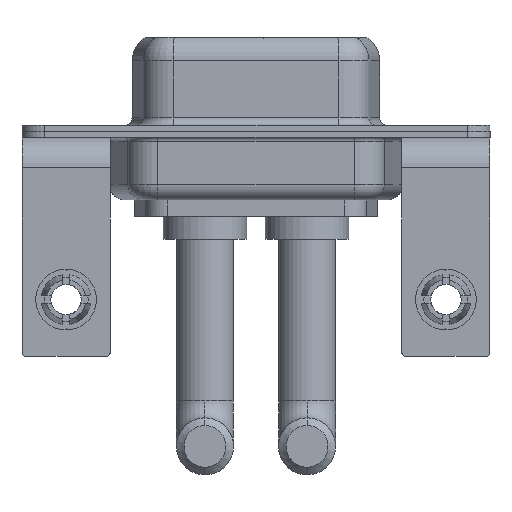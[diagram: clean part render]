
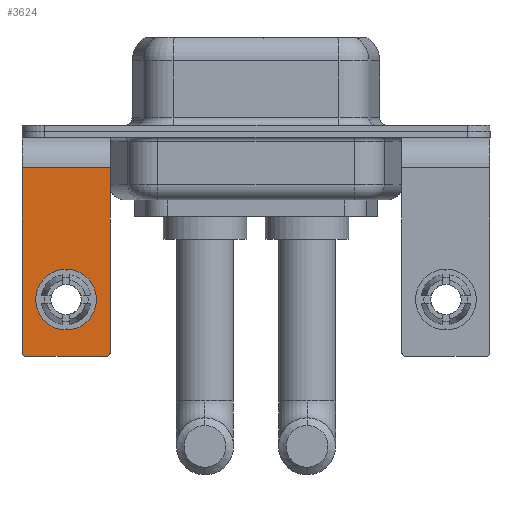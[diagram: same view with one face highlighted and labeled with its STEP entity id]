
A CAD part, front view. The second image highlights one B-rep face of the part: STEP entity #3624.
In plain terms, the highlighted planar face has unit normal (0, -1, 0).
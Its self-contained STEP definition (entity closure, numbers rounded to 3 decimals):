
#23 = DIRECTION ( 'NONE',  ( 0., 0., 1. ) ) ;
#254 = ORIENTED_EDGE ( 'NONE', *, *, #11016, .T. ) ;
#834 = CARTESIAN_POINT ( 'NONE',  ( 2.9, -6.25, -2.4 ) ) ;
#1071 = DIRECTION ( 'NONE',  ( 0., 1., 0. ) ) ;
#1249 = CARTESIAN_POINT ( 'NONE',  ( 2.65, -6.25, -14.8 ) ) ;
#1402 = CARTESIAN_POINT ( 'NONE',  ( -2.9, -6.25, -14.55 ) ) ;
#1406 = EDGE_CURVE ( 'NONE', #9233, #6474, #4739, .T. ) ;
#2445 = ORIENTED_EDGE ( 'NONE', *, *, #6453, .T. ) ;
#2625 = DIRECTION ( 'NONE',  ( 0., -1., 0. ) ) ;
#2929 = CARTESIAN_POINT ( 'NONE',  ( 0., -6.25, -11.07 ) ) ;
#3060 = CARTESIAN_POINT ( 'NONE',  ( 2.9, -6.25, -14.55 ) ) ;
#3472 = ORIENTED_EDGE ( 'NONE', *, *, #8617, .T. ) ;
#3624 = ADVANCED_FACE ( 'NONE', ( #4878, #4643 ), #10825, .F. ) ;
#3916 = DIRECTION ( 'NONE',  ( 0., 1., 0. ) ) ;
#4448 = ORIENTED_EDGE ( 'NONE', *, *, #8715, .T. ) ;
#4521 = VERTEX_POINT ( 'NONE', #1402 ) ;
#4624 = EDGE_CURVE ( 'NONE', #6474, #9233, #7507, .T. ) ;
#4631 = CARTESIAN_POINT ( 'NONE',  ( 2.65, -6.25, -14.55 ) ) ;
#4643 = FACE_OUTER_BOUND ( 'NONE', #7468, .T. ) ;
#4739 = CIRCLE ( 'NONE', #14375, 2. ) ;
#4878 = FACE_BOUND ( 'NONE', #11897, .T. ) ;
#5662 = EDGE_CURVE ( 'NONE', #8594, #13897, #6390, .T. ) ;
#6112 = AXIS2_PLACEMENT_3D ( 'NONE', #14547, #2625, #23 ) ;
#6349 = VERTEX_POINT ( 'NONE', #1249 ) ;
#6390 = LINE ( 'NONE', #8855, #10854 ) ;
#6453 = EDGE_CURVE ( 'NONE', #6846, #4521, #7923, .T. ) ;
#6474 = VERTEX_POINT ( 'NONE', #8875 ) ;
#6846 = VERTEX_POINT ( 'NONE', #13601 ) ;
#7468 = EDGE_LOOP ( 'NONE', ( #2445, #4448, #9600, #3472, #8025, #254 ) ) ;
#7507 = CIRCLE ( 'NONE', #9537, 2. ) ;
#7571 = DIRECTION ( 'NONE',  ( 0., 1., 0. ) ) ;
#7827 = CARTESIAN_POINT ( 'NONE',  ( 0., -6.25, -11.07 ) ) ;
#7923 = LINE ( 'NONE', #10120, #14914 ) ;
#8025 = ORIENTED_EDGE ( 'NONE', *, *, #5662, .F. ) ;
#8559 = VERTEX_POINT ( 'NONE', #10661 ) ;
#8594 = VERTEX_POINT ( 'NONE', #834 ) ;
#8617 = EDGE_CURVE ( 'NONE', #6349, #13897, #9399, .T. ) ;
#8656 = CIRCLE ( 'NONE', #6112, 0.25 ) ;
#8715 = EDGE_CURVE ( 'NONE', #4521, #8559, #8656, .T. ) ;
#8855 = CARTESIAN_POINT ( 'NONE',  ( 2.9, -6.25, -2.4 ) ) ;
#8875 = CARTESIAN_POINT ( 'NONE',  ( 0., -6.25, -13.07 ) ) ;
#8977 = EDGE_CURVE ( 'NONE', #6349, #8559, #12467, .T. ) ;
#9154 = CARTESIAN_POINT ( 'NONE',  ( 2.9, -6.25, -14.8 ) ) ;
#9233 = VERTEX_POINT ( 'NONE', #12062 ) ;
#9399 = CIRCLE ( 'NONE', #11400, 0.25 ) ;
#9537 = AXIS2_PLACEMENT_3D ( 'NONE', #2929, #7571, #11349 ) ;
#9569 = CARTESIAN_POINT ( 'NONE',  ( 2.9, -6.25, -2.4 ) ) ;
#9600 = ORIENTED_EDGE ( 'NONE', *, *, #8977, .F. ) ;
#10110 = DIRECTION ( 'NONE',  ( 0., 0., 1. ) ) ;
#10120 = CARTESIAN_POINT ( 'NONE',  ( -2.9, -6.25, -2.4 ) ) ;
#10504 = DIRECTION ( 'NONE',  ( 0., 0., 1. ) ) ;
#10562 = AXIS2_PLACEMENT_3D ( 'NONE', #9569, #1071, #12167 ) ;
#10661 = CARTESIAN_POINT ( 'NONE',  ( -2.65, -6.25, -14.8 ) ) ;
#10825 = PLANE ( 'NONE',  #10562 ) ;
#10854 = VECTOR ( 'NONE', #13835, 1000. ) ;
#11016 = EDGE_CURVE ( 'NONE', #8594, #6846, #14333, .T. ) ;
#11349 = DIRECTION ( 'NONE',  ( 0., 0., 1. ) ) ;
#11400 = AXIS2_PLACEMENT_3D ( 'NONE', #4631, #14239, #10504 ) ;
#11538 = VECTOR ( 'NONE', #13287, 1000. ) ;
#11897 = EDGE_LOOP ( 'NONE', ( #12176, #15082 ) ) ;
#11912 = VECTOR ( 'NONE', #13740, 1000. ) ;
#12014 = CARTESIAN_POINT ( 'NONE',  ( 2.9, -6.25, -2.4 ) ) ;
#12062 = CARTESIAN_POINT ( 'NONE',  ( 0., -6.25, -9.07 ) ) ;
#12167 = DIRECTION ( 'NONE',  ( 0., 0., 1. ) ) ;
#12176 = ORIENTED_EDGE ( 'NONE', *, *, #4624, .T. ) ;
#12467 = LINE ( 'NONE', #9154, #11912 ) ;
#12501 = DIRECTION ( 'NONE',  ( 0., 0., -1. ) ) ;
#13287 = DIRECTION ( 'NONE',  ( -1., 0., 0. ) ) ;
#13601 = CARTESIAN_POINT ( 'NONE',  ( -2.9, -6.25, -2.4 ) ) ;
#13740 = DIRECTION ( 'NONE',  ( -1., 0., 0. ) ) ;
#13835 = DIRECTION ( 'NONE',  ( 0., 0., -1. ) ) ;
#13897 = VERTEX_POINT ( 'NONE', #3060 ) ;
#14239 = DIRECTION ( 'NONE',  ( 0., -1., 0. ) ) ;
#14333 = LINE ( 'NONE', #12014, #11538 ) ;
#14375 = AXIS2_PLACEMENT_3D ( 'NONE', #7827, #3916, #10110 ) ;
#14547 = CARTESIAN_POINT ( 'NONE',  ( -2.65, -6.25, -14.55 ) ) ;
#14914 = VECTOR ( 'NONE', #12501, 1000. ) ;
#15082 = ORIENTED_EDGE ( 'NONE', *, *, #1406, .T. ) ;
